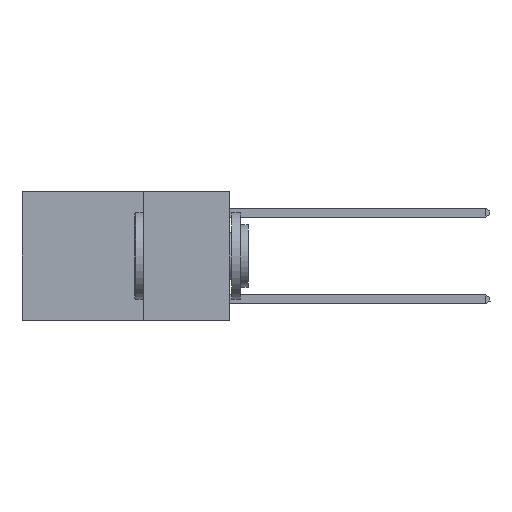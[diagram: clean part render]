
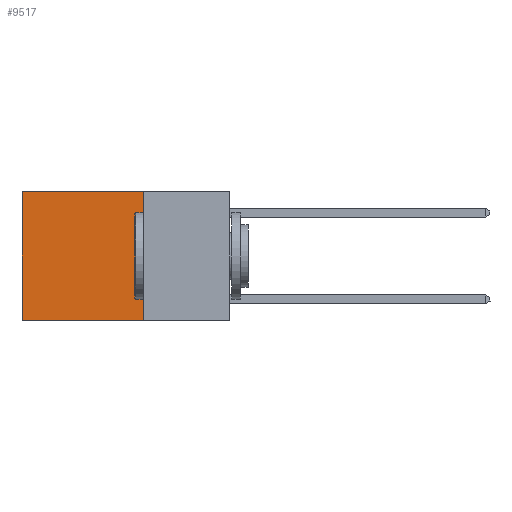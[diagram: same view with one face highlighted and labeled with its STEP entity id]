
A CAD part, left-side view. The second image highlights one B-rep face of the part: STEP entity #9517.
In plain terms, the highlighted planar face has unit normal (-1, 0, 0).
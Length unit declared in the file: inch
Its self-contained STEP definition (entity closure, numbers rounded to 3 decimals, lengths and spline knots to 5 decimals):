
#314 = EDGE_CURVE ( 'NONE', #19768, #10618, #9012, .T. ) ;
#1122 = DIRECTION ( 'NONE',  ( 0., 1., 0. ) ) ;
#2184 = CARTESIAN_POINT ( 'NONE',  ( 0.2625, 0.25, -0.37 ) ) ;
#2238 = CARTESIAN_POINT ( 'NONE',  ( 0.2625, 0.6, -0.37 ) ) ;
#3141 = FACE_OUTER_BOUND ( 'NONE', #9072, .T. ) ;
#3190 = DIRECTION ( 'NONE',  ( 1., 0., 0. ) ) ;
#3574 = VERTEX_POINT ( 'NONE', #9538 ) ;
#3812 = LINE ( 'NONE', #17091, #5380 ) ;
#4541 = LINE ( 'NONE', #11088, #19514 ) ;
#5123 = LINE ( 'NONE', #2184, #6700 ) ;
#5380 = VECTOR ( 'NONE', #10556, 39.37008 ) ;
#5601 = CARTESIAN_POINT ( 'NONE',  ( 0.2625, 0.25, 0. ) ) ;
#5691 = DIRECTION ( 'NONE',  ( 0., 1., 0. ) ) ;
#6700 = VECTOR ( 'NONE', #5691, 39.37008 ) ;
#6816 = EDGE_CURVE ( 'NONE', #10618, #7379, #5123, .T. ) ;
#6842 = CARTESIAN_POINT ( 'NONE',  ( 0.2625, 0.25, 0. ) ) ;
#7328 = DIRECTION ( 'NONE',  ( 0., 0., -1. ) ) ;
#7379 = VERTEX_POINT ( 'NONE', #2238 ) ;
#8132 = EDGE_CURVE ( 'NONE', #19768, #3574, #4541, .T. ) ;
#8510 = DIRECTION ( 'NONE',  ( 0., 0., -1. ) ) ;
#9012 = LINE ( 'NONE', #5601, #19061 ) ;
#9072 = EDGE_LOOP ( 'NONE', ( #18636, #19791, #20828, #11307 ) ) ;
#9517 = ADVANCED_FACE ( 'NONE', ( #3141 ), #16717, .F. ) ;
#9538 = CARTESIAN_POINT ( 'NONE',  ( 0.2625, 0.6, 0. ) ) ;
#10556 = DIRECTION ( 'NONE',  ( 0., 0., -1. ) ) ;
#10618 = VERTEX_POINT ( 'NONE', #20840 ) ;
#11088 = CARTESIAN_POINT ( 'NONE',  ( 0.2625, 0.25, 0. ) ) ;
#11307 = ORIENTED_EDGE ( 'NONE', *, *, #8132, .T. ) ;
#11565 = AXIS2_PLACEMENT_3D ( 'NONE', #6842, #3190, #8510 ) ;
#12053 = CARTESIAN_POINT ( 'NONE',  ( 0.2625, 0.25, 0. ) ) ;
#12152 = EDGE_CURVE ( 'NONE', #3574, #7379, #3812, .T. ) ;
#16717 = PLANE ( 'NONE',  #11565 ) ;
#17091 = CARTESIAN_POINT ( 'NONE',  ( 0.2625, 0.6, 0. ) ) ;
#18636 = ORIENTED_EDGE ( 'NONE', *, *, #12152, .T. ) ;
#19061 = VECTOR ( 'NONE', #7328, 39.37008 ) ;
#19514 = VECTOR ( 'NONE', #1122, 39.37008 ) ;
#19768 = VERTEX_POINT ( 'NONE', #12053 ) ;
#19791 = ORIENTED_EDGE ( 'NONE', *, *, #6816, .F. ) ;
#20828 = ORIENTED_EDGE ( 'NONE', *, *, #314, .F. ) ;
#20840 = CARTESIAN_POINT ( 'NONE',  ( 0.2625, 0.25, -0.37 ) ) ;
